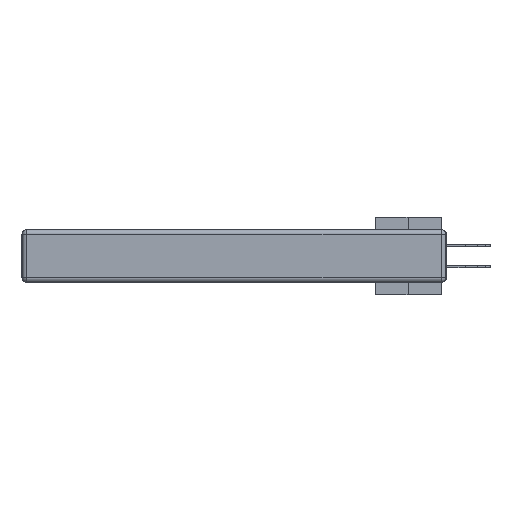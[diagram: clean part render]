
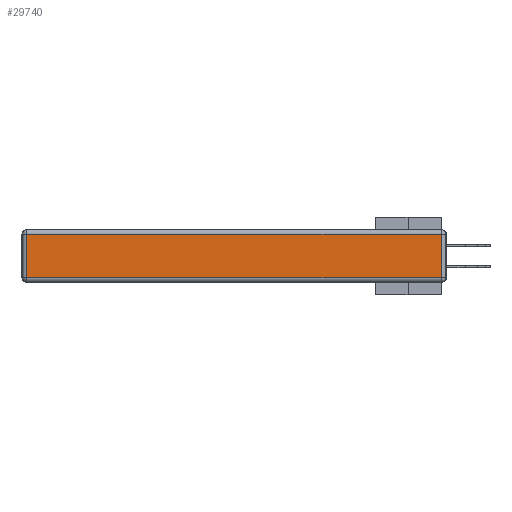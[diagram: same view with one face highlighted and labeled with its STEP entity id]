
A CAD part, left-side view. The second image highlights one B-rep face of the part: STEP entity #29740.
In plain terms, the highlighted planar face has unit normal (-1, 0, 0).
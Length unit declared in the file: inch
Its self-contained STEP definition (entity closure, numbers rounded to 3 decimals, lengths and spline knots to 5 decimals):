
#913 = VECTOR ( 'NONE', #11147, 39.37008 ) ;
#1190 = VECTOR ( 'NONE', #17292, 39.37008 ) ;
#1463 = CARTESIAN_POINT ( 'NONE',  ( 0., 0.03, -0.313 ) ) ;
#2729 = LINE ( 'NONE', #14202, #1190 ) ;
#7632 = DIRECTION ( 'NONE',  ( -1., 0., 0. ) ) ;
#10277 = VERTEX_POINT ( 'NONE', #1463 ) ;
#10575 = PLANE ( 'NONE',  #33313 ) ;
#11147 = DIRECTION ( 'NONE',  ( 0., -1., 0. ) ) ;
#13057 = EDGE_CURVE ( 'NONE', #42967, #16571, #2729, .T. ) ;
#14202 = CARTESIAN_POINT ( 'NONE',  ( 0., 2.72, -0.343 ) ) ;
#14203 = CARTESIAN_POINT ( 'NONE',  ( 0., 0., -0.313 ) ) ;
#16571 = VERTEX_POINT ( 'NONE', #25859 ) ;
#16629 = DIRECTION ( 'NONE',  ( 0., 0., 1. ) ) ;
#16674 = ORIENTED_EDGE ( 'NONE', *, *, #13057, .T. ) ;
#16748 = ORIENTED_EDGE ( 'NONE', *, *, #19116, .T. ) ;
#17279 = CARTESIAN_POINT ( 'NONE',  ( 0., 0., -0.343 ) ) ;
#17292 = DIRECTION ( 'NONE',  ( 0., 0., -1. ) ) ;
#18708 = LINE ( 'NONE', #14203, #913 ) ;
#19116 = EDGE_CURVE ( 'NONE', #10277, #23940, #39295, .T. ) ;
#21071 = DIRECTION ( 'NONE',  ( 0., 0., 1. ) ) ;
#22876 = CARTESIAN_POINT ( 'NONE',  ( 0., 0.03, -0.03 ) ) ;
#23940 = VERTEX_POINT ( 'NONE', #22876 ) ;
#23982 = ORIENTED_EDGE ( 'NONE', *, *, #39243, .T. ) ;
#24322 = EDGE_LOOP ( 'NONE', ( #23982, #16748, #40039, #16674 ) ) ;
#25859 = CARTESIAN_POINT ( 'NONE',  ( 0., 2.72, -0.313 ) ) ;
#26870 = CARTESIAN_POINT ( 'NONE',  ( 0., 0.03, -0.343 ) ) ;
#27788 = VECTOR ( 'NONE', #16629, 39.37008 ) ;
#29179 = EDGE_CURVE ( 'NONE', #23940, #42967, #42705, .T. ) ;
#29740 = ADVANCED_FACE ( 'NONE', ( #33794 ), #10575, .T. ) ;
#29882 = DIRECTION ( 'NONE',  ( 0., 1., 0. ) ) ;
#30183 = CARTESIAN_POINT ( 'NONE',  ( 0., 2.75, -0.03 ) ) ;
#30384 = CARTESIAN_POINT ( 'NONE',  ( 0., 2.72, -0.03 ) ) ;
#33313 = AXIS2_PLACEMENT_3D ( 'NONE', #17279, #7632, #21071 ) ;
#33794 = FACE_OUTER_BOUND ( 'NONE', #24322, .T. ) ;
#39243 = EDGE_CURVE ( 'NONE', #16571, #10277, #18708, .T. ) ;
#39295 = LINE ( 'NONE', #26870, #27788 ) ;
#39559 = VECTOR ( 'NONE', #29882, 39.37008 ) ;
#40039 = ORIENTED_EDGE ( 'NONE', *, *, #29179, .T. ) ;
#42705 = LINE ( 'NONE', #30183, #39559 ) ;
#42967 = VERTEX_POINT ( 'NONE', #30384 ) ;
